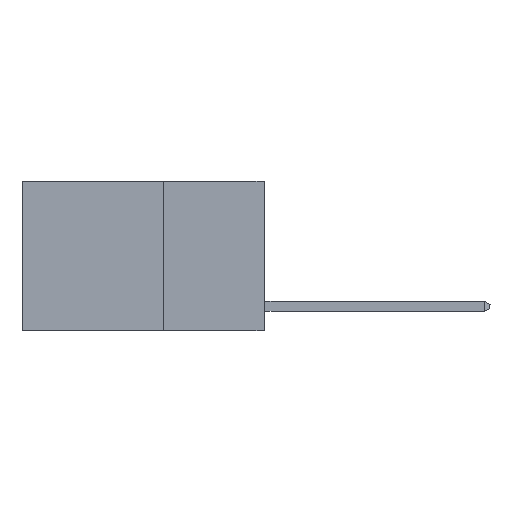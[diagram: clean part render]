
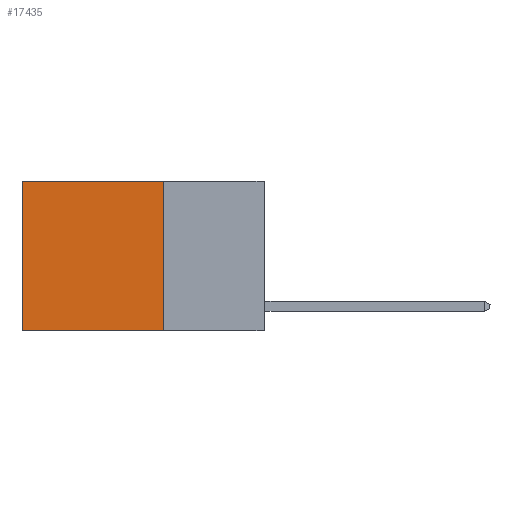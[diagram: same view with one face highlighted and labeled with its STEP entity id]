
A CAD part, left-side view. The second image highlights one B-rep face of the part: STEP entity #17435.
In plain terms, the highlighted planar face has unit normal (-1, 0, 0).
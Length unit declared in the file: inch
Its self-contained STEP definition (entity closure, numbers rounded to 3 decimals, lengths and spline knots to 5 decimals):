
#436 = ORIENTED_EDGE ( 'NONE', *, *, #8528, .T. ) ;
#1487 = LINE ( 'NONE', #12758, #17382 ) ;
#1764 = VERTEX_POINT ( 'NONE', #9843 ) ;
#2177 = EDGE_CURVE ( 'NONE', #1764, #11200, #1487, .T. ) ;
#2855 = ORIENTED_EDGE ( 'NONE', *, *, #4027, .T. ) ;
#3436 = DIRECTION ( 'NONE',  ( 1., 0., 0. ) ) ;
#4027 = EDGE_CURVE ( 'NONE', #15886, #17098, #8821, .T. ) ;
#4797 = CARTESIAN_POINT ( 'NONE',  ( 0.2625, 0.25, 0. ) ) ;
#5310 = ORIENTED_EDGE ( 'NONE', *, *, #2177, .F. ) ;
#5657 = CARTESIAN_POINT ( 'NONE',  ( 0.2625, 0.6, -0.37 ) ) ;
#5801 = DIRECTION ( 'NONE',  ( 0., 1., 0. ) ) ;
#6118 = VECTOR ( 'NONE', #18524, 39.37008 ) ;
#7313 = VECTOR ( 'NONE', #17254, 39.37008 ) ;
#7826 = EDGE_LOOP ( 'NONE', ( #436, #5310, #21674, #2855 ) ) ;
#8528 = EDGE_CURVE ( 'NONE', #17098, #11200, #18161, .T. ) ;
#8821 = LINE ( 'NONE', #15158, #21556 ) ;
#9843 = CARTESIAN_POINT ( 'NONE',  ( 0.2625, 0.25, -0.37 ) ) ;
#10724 = DIRECTION ( 'NONE',  ( 0., 1., 0. ) ) ;
#11200 = VERTEX_POINT ( 'NONE', #5657 ) ;
#11406 = EDGE_CURVE ( 'NONE', #15886, #1764, #19614, .T. ) ;
#11525 = AXIS2_PLACEMENT_3D ( 'NONE', #20112, #3436, #20338 ) ;
#12142 = CARTESIAN_POINT ( 'NONE',  ( 0.2625, 0.6, 0. ) ) ;
#12710 = FACE_OUTER_BOUND ( 'NONE', #7826, .T. ) ;
#12758 = CARTESIAN_POINT ( 'NONE',  ( 0.2625, 0.25, -0.37 ) ) ;
#13471 = PLANE ( 'NONE',  #11525 ) ;
#15158 = CARTESIAN_POINT ( 'NONE',  ( 0.2625, 0.25, 0. ) ) ;
#15886 = VERTEX_POINT ( 'NONE', #20549 ) ;
#16161 = CARTESIAN_POINT ( 'NONE',  ( 0.2625, 0.6, 0. ) ) ;
#17098 = VERTEX_POINT ( 'NONE', #16161 ) ;
#17254 = DIRECTION ( 'NONE',  ( 0., 0., -1. ) ) ;
#17382 = VECTOR ( 'NONE', #5801, 39.37008 ) ;
#17435 = ADVANCED_FACE ( 'NONE', ( #12710 ), #13471, .F. ) ;
#18161 = LINE ( 'NONE', #12142, #7313 ) ;
#18524 = DIRECTION ( 'NONE',  ( 0., 0., -1. ) ) ;
#19614 = LINE ( 'NONE', #4797, #6118 ) ;
#20112 = CARTESIAN_POINT ( 'NONE',  ( 0.2625, 0.25, 0. ) ) ;
#20338 = DIRECTION ( 'NONE',  ( 0., 0., -1. ) ) ;
#20549 = CARTESIAN_POINT ( 'NONE',  ( 0.2625, 0.25, 0. ) ) ;
#21556 = VECTOR ( 'NONE', #10724, 39.37008 ) ;
#21674 = ORIENTED_EDGE ( 'NONE', *, *, #11406, .F. ) ;
